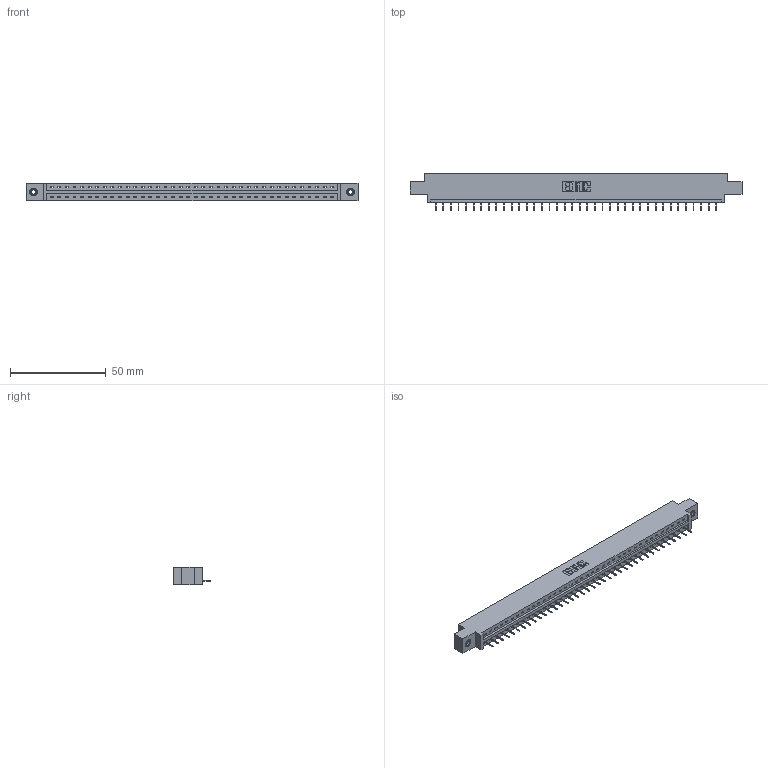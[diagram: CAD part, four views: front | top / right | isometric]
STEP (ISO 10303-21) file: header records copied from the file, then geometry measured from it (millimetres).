
FILE_DESCRIPTION (( 'STEP AP203' ), '1' );
FILE_NAME ('387-038-524-608.STEP', '2018-09-19T04:43:19', ( '' ), ( '' ), 'SwSTEP 2.0', 'SolidWorks 2016', '' );
FILE_SCHEMA (( 'CONFIG_CONTROL_DESIGN' ));
Length unit declared in the file: inch
Products named in the file (4): 337 Part_0.170 Offset - 0.156 Dia-TI; 345-292-001_345-293-124; 345-250-001_345-250-003-102; 387-038-524-608
Assembly tree (41 placements, depth 2):
  387-038-524-608
    337 Part_0.170 Offset - 0.156 Dia-TI
    345-292-001_345-293-124  x38
    345-250-001_345-250-003-102  x2
Bounding box: 173.58 x 19.69 x 9.4 mm (x, y, z)
Volume: 17716.9 mm3; surface area: 17883.9 mm2
Topology: 41 solids, 41 shells, 2686 faces, 7755 edges, 5010 vertices
Faces by surface type: plane 2082, cylinder 588, cone 12, torus 4
Entity records: 30156 total; most frequent: CARTESIAN_POINT 5231, ORIENTED_EDGE 5198, DIRECTION 4445, EDGE_CURVE 2599, LINE 2455, VECTOR 2455, VERTEX_POINT 1724, AXIS2_PLACEMENT_3D 995
